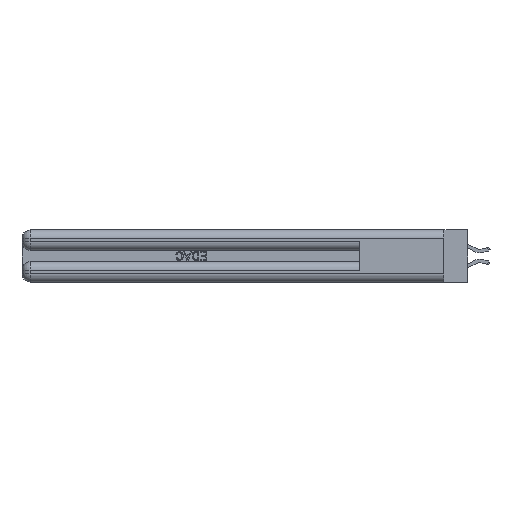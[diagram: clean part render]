
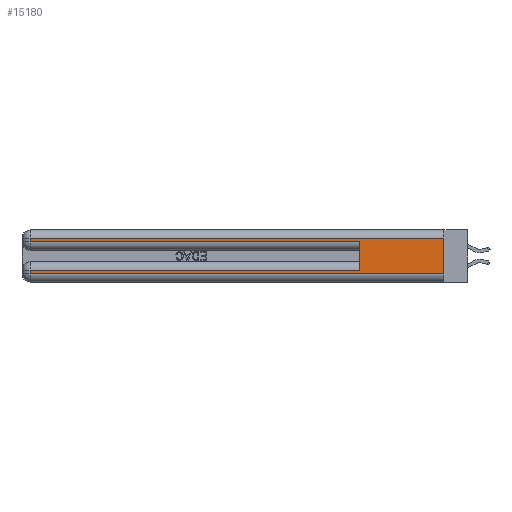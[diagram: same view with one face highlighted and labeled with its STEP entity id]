
A CAD part, left-side view. The second image highlights one B-rep face of the part: STEP entity #15180.
In plain terms, the highlighted planar face has unit normal (-1, 0, 0).
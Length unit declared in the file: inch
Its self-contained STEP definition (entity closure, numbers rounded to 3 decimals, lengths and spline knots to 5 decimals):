
#150 = VECTOR ( 'NONE', #22464, 39.37008 ) ;
#2081 = VERTEX_POINT ( 'NONE', #21682 ) ;
#2165 = EDGE_CURVE ( 'NONE', #2081, #39957, #3882, .T. ) ;
#3281 = CARTESIAN_POINT ( 'NONE',  ( 0., 2.94, 0.37 ) ) ;
#3482 = DIRECTION ( 'NONE',  ( 0., 1., 0. ) ) ;
#3882 = LINE ( 'NONE', #14593, #30457 ) ;
#4465 = LINE ( 'NONE', #35790, #41860 ) ;
#6002 = CARTESIAN_POINT ( 'NONE',  ( 0., 0.6, 0.145 ) ) ;
#6216 = ORIENTED_EDGE ( 'NONE', *, *, #36186, .T. ) ;
#6223 = CARTESIAN_POINT ( 'NONE',  ( 0., 0., 0.06 ) ) ;
#6407 = LINE ( 'NONE', #3281, #21136 ) ;
#6572 = VECTOR ( 'NONE', #3482, 39.37008 ) ;
#6716 = VERTEX_POINT ( 'NONE', #46017 ) ;
#7429 = EDGE_CURVE ( 'NONE', #39957, #6716, #30466, .T. ) ;
#7763 = PLANE ( 'NONE',  #25212 ) ;
#8520 = DIRECTION ( 'NONE',  ( 0., 0., -1. ) ) ;
#8806 = VECTOR ( 'NONE', #38735, 39.37008 ) ;
#11722 = VECTOR ( 'NONE', #33088, 39.37008 ) ;
#13680 = ORIENTED_EDGE ( 'NONE', *, *, #43003, .F. ) ;
#14593 = CARTESIAN_POINT ( 'NONE',  ( 0., 0., 0.31 ) ) ;
#14643 = CARTESIAN_POINT ( 'NONE',  ( 0., 2.94, 0.085 ) ) ;
#15043 = VERTEX_POINT ( 'NONE', #30994 ) ;
#15107 = DIRECTION ( 'NONE',  ( 1., 0., 0. ) ) ;
#15180 = ADVANCED_FACE ( 'NONE', ( #26293 ), #7763, .F. ) ;
#15749 = ORIENTED_EDGE ( 'NONE', *, *, #20489, .T. ) ;
#16260 = LINE ( 'NONE', #6002, #8806 ) ;
#16420 = VECTOR ( 'NONE', #8520, 39.37008 ) ;
#16429 = EDGE_CURVE ( 'NONE', #2081, #34569, #33560, .T. ) ;
#18754 = DIRECTION ( 'NONE',  ( 0., 0., -1. ) ) ;
#20489 = EDGE_CURVE ( 'NONE', #41147, #46711, #24680, .T. ) ;
#21136 = VECTOR ( 'NONE', #35821, 39.37008 ) ;
#21682 = CARTESIAN_POINT ( 'NONE',  ( 0., 0., 0.31 ) ) ;
#22464 = DIRECTION ( 'NONE',  ( 0., 0., -1. ) ) ;
#22528 = CARTESIAN_POINT ( 'NONE',  ( 0., 0., 0.285 ) ) ;
#23021 = CARTESIAN_POINT ( 'NONE',  ( 0., 2.94, 0.31 ) ) ;
#24211 = LINE ( 'NONE', #22528, #11722 ) ;
#24543 = ORIENTED_EDGE ( 'NONE', *, *, #2165, .T. ) ;
#24615 = DIRECTION ( 'NONE',  ( 0., -1., 0. ) ) ;
#24653 = ORIENTED_EDGE ( 'NONE', *, *, #16429, .F. ) ;
#24680 = LINE ( 'NONE', #46283, #6572 ) ;
#25212 = AXIS2_PLACEMENT_3D ( 'NONE', #33058, #15107, #18754 ) ;
#26293 = FACE_OUTER_BOUND ( 'NONE', #32277, .T. ) ;
#29499 = CARTESIAN_POINT ( 'NONE',  ( 0., 0.6, 0.085 ) ) ;
#30457 = VECTOR ( 'NONE', #36313, 39.37008 ) ;
#30466 = LINE ( 'NONE', #45449, #16420 ) ;
#30994 = CARTESIAN_POINT ( 'NONE',  ( 0., 0.6, 0.285 ) ) ;
#32277 = EDGE_LOOP ( 'NONE', ( #24653, #24543, #37100, #6216, #13680, #15749, #40095, #40308 ) ) ;
#33058 = CARTESIAN_POINT ( 'NONE',  ( 0., 0., 0.37 ) ) ;
#33088 = DIRECTION ( 'NONE',  ( 0., -1., 0. ) ) ;
#33560 = LINE ( 'NONE', #36797, #150 ) ;
#34569 = VERTEX_POINT ( 'NONE', #6223 ) ;
#35790 = CARTESIAN_POINT ( 'NONE',  ( 0., 0., 0.06 ) ) ;
#35821 = DIRECTION ( 'NONE',  ( 0., 0., -1. ) ) ;
#36186 = EDGE_CURVE ( 'NONE', #6716, #15043, #24211, .T. ) ;
#36313 = DIRECTION ( 'NONE',  ( 0., 1., 0. ) ) ;
#36797 = CARTESIAN_POINT ( 'NONE',  ( 0., 0., 0.37 ) ) ;
#37100 = ORIENTED_EDGE ( 'NONE', *, *, #7429, .T. ) ;
#38735 = DIRECTION ( 'NONE',  ( 0., 0., 1. ) ) ;
#38799 = EDGE_CURVE ( 'NONE', #46711, #43849, #6407, .T. ) ;
#39957 = VERTEX_POINT ( 'NONE', #23021 ) ;
#40095 = ORIENTED_EDGE ( 'NONE', *, *, #38799, .T. ) ;
#40110 = CARTESIAN_POINT ( 'NONE',  ( 0., 2.94, 0.06 ) ) ;
#40308 = ORIENTED_EDGE ( 'NONE', *, *, #41419, .T. ) ;
#41147 = VERTEX_POINT ( 'NONE', #29499 ) ;
#41419 = EDGE_CURVE ( 'NONE', #43849, #34569, #4465, .T. ) ;
#41860 = VECTOR ( 'NONE', #24615, 39.37008 ) ;
#43003 = EDGE_CURVE ( 'NONE', #41147, #15043, #16260, .T. ) ;
#43849 = VERTEX_POINT ( 'NONE', #40110 ) ;
#45449 = CARTESIAN_POINT ( 'NONE',  ( 0., 2.94, 0.37 ) ) ;
#46017 = CARTESIAN_POINT ( 'NONE',  ( 0., 2.94, 0.285 ) ) ;
#46283 = CARTESIAN_POINT ( 'NONE',  ( 0., 0., 0.085 ) ) ;
#46711 = VERTEX_POINT ( 'NONE', #14643 ) ;
